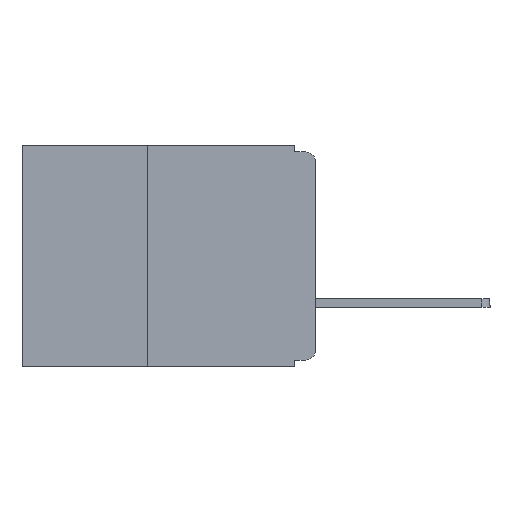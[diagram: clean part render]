
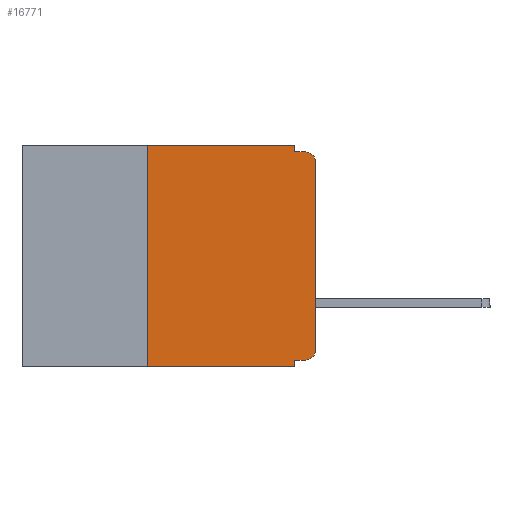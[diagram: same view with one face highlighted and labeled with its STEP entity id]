
A CAD part, left-side view. The second image highlights one B-rep face of the part: STEP entity #16771.
In plain terms, the highlighted planar face has unit normal (-1, 0, 0).
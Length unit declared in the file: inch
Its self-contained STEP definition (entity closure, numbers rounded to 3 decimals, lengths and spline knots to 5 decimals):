
#26 = PLANE ( 'NONE',  #10962 ) ;
#110 = CARTESIAN_POINT ( 'NONE',  ( 0., 0.437, 0. ) ) ;
#758 = ORIENTED_EDGE ( 'NONE', *, *, #4400, .T. ) ;
#957 = CARTESIAN_POINT ( 'NONE',  ( 0., 0., -0.305 ) ) ;
#1059 = CARTESIAN_POINT ( 'NONE',  ( 0., 0.031, 0. ) ) ;
#1191 = DIRECTION ( 'NONE',  ( 0., 0., -1. ) ) ;
#1295 = ORIENTED_EDGE ( 'NONE', *, *, #5879, .F. ) ;
#1357 = VERTEX_POINT ( 'NONE', #16873 ) ;
#1403 = VECTOR ( 'NONE', #18997, 39.37008 ) ;
#1561 = LINE ( 'NONE', #16957, #1403 ) ;
#1664 = VECTOR ( 'NONE', #6041, 39.37008 ) ;
#1813 = CARTESIAN_POINT ( 'NONE',  ( 0., 0.25, 0. ) ) ;
#1842 = LINE ( 'NONE', #18435, #1664 ) ;
#1916 = VERTEX_POINT ( 'NONE', #14373 ) ;
#2876 = VERTEX_POINT ( 'NONE', #17773 ) ;
#3123 = CARTESIAN_POINT ( 'NONE',  ( 0., 0.015, -0.32 ) ) ;
#3374 = DIRECTION ( 'NONE',  ( 0., 1., 0. ) ) ;
#3438 = CARTESIAN_POINT ( 'NONE',  ( 0., 0.25, -0.33 ) ) ;
#3558 = FACE_OUTER_BOUND ( 'NONE', #6465, .T. ) ;
#3839 = CARTESIAN_POINT ( 'NONE',  ( 0., 0., -0.32 ) ) ;
#3941 = CIRCLE ( 'NONE', #15819, 0.015 ) ;
#4025 = VECTOR ( 'NONE', #5223, 39.37008 ) ;
#4045 = LINE ( 'NONE', #4946, #4025 ) ;
#4400 = EDGE_CURVE ( 'NONE', #10610, #18652, #4756, .T. ) ;
#4712 = VECTOR ( 'NONE', #15009, 39.37008 ) ;
#4756 = LINE ( 'NONE', #14314, #4712 ) ;
#4854 = VECTOR ( 'NONE', #18071, 39.37008 ) ;
#4946 = CARTESIAN_POINT ( 'NONE',  ( 0., 0., -0.01 ) ) ;
#4978 = ORIENTED_EDGE ( 'NONE', *, *, #18513, .T. ) ;
#5032 = LINE ( 'NONE', #17976, #4854 ) ;
#5223 = DIRECTION ( 'NONE',  ( 0., -1., 0. ) ) ;
#5879 = EDGE_CURVE ( 'NONE', #12485, #2876, #12464, .T. ) ;
#6041 = DIRECTION ( 'NONE',  ( 0., -1., 0. ) ) ;
#6465 = EDGE_LOOP ( 'NONE', ( #758, #8889, #9563, #11610, #12666, #15090, #16672, #1295, #12717, #4978 ) ) ;
#7396 = VECTOR ( 'NONE', #3374, 39.37008 ) ;
#7537 = LINE ( 'NONE', #3839, #7396 ) ;
#7982 = CIRCLE ( 'NONE', #18578, 0.015 ) ;
#8578 = VECTOR ( 'NONE', #16058, 39.37008 ) ;
#8889 = ORIENTED_EDGE ( 'NONE', *, *, #14869, .T. ) ;
#9548 = DIRECTION ( 'NONE',  ( 0., 0., -1. ) ) ;
#9563 = ORIENTED_EDGE ( 'NONE', *, *, #11146, .F. ) ;
#9613 = DIRECTION ( 'NONE',  ( -1., 0., 0. ) ) ;
#9686 = CARTESIAN_POINT ( 'NONE',  ( 0., 0.015, -0.025 ) ) ;
#9831 = VERTEX_POINT ( 'NONE', #14413 ) ;
#10332 = EDGE_CURVE ( 'NONE', #17789, #2876, #1842, .T. ) ;
#10610 = VERTEX_POINT ( 'NONE', #957 ) ;
#10962 = AXIS2_PLACEMENT_3D ( 'NONE', #110, #19120, #19111 ) ;
#11146 = EDGE_CURVE ( 'NONE', #1357, #9831, #4045, .T. ) ;
#11537 = VERTEX_POINT ( 'NONE', #1813 ) ;
#11610 = ORIENTED_EDGE ( 'NONE', *, *, #17842, .F. ) ;
#11834 = CARTESIAN_POINT ( 'NONE',  ( 0., 0.031, -0.32 ) ) ;
#12326 = VECTOR ( 'NONE', #1191, 39.37008 ) ;
#12401 = LINE ( 'NONE', #1059, #12326 ) ;
#12464 = LINE ( 'NONE', #16303, #8578 ) ;
#12485 = VERTEX_POINT ( 'NONE', #11834 ) ;
#12666 = ORIENTED_EDGE ( 'NONE', *, *, #19063, .F. ) ;
#12717 = ORIENTED_EDGE ( 'NONE', *, *, #18622, .F. ) ;
#14314 = CARTESIAN_POINT ( 'NONE',  ( 0., 0., 0. ) ) ;
#14373 = CARTESIAN_POINT ( 'NONE',  ( 0., 0.031, 0. ) ) ;
#14413 = CARTESIAN_POINT ( 'NONE',  ( 0., 0.015, -0.01 ) ) ;
#14869 = EDGE_CURVE ( 'NONE', #18652, #9831, #3941, .T. ) ;
#15009 = DIRECTION ( 'NONE',  ( 0., 0., 1. ) ) ;
#15090 = ORIENTED_EDGE ( 'NONE', *, *, #17062, .F. ) ;
#15819 = AXIS2_PLACEMENT_3D ( 'NONE', #9686, #9613, #9548 ) ;
#15890 = DIRECTION ( 'NONE',  ( 0., 0., -1. ) ) ;
#16058 = DIRECTION ( 'NONE',  ( 0., 0., -1. ) ) ;
#16303 = CARTESIAN_POINT ( 'NONE',  ( 0., 0.031, -0.33 ) ) ;
#16672 = ORIENTED_EDGE ( 'NONE', *, *, #10332, .T. ) ;
#16714 = VERTEX_POINT ( 'NONE', #3123 ) ;
#16771 = ADVANCED_FACE ( 'NONE', ( #3558 ), #26, .F. ) ;
#16873 = CARTESIAN_POINT ( 'NONE',  ( 0., 0.031, -0.01 ) ) ;
#16939 = DIRECTION ( 'NONE',  ( -1., 0., 0. ) ) ;
#16957 = CARTESIAN_POINT ( 'NONE',  ( 0., 0.25, -0.33 ) ) ;
#16987 = CARTESIAN_POINT ( 'NONE',  ( 0., 0.015, -0.305 ) ) ;
#17062 = EDGE_CURVE ( 'NONE', #17789, #11537, #1561, .T. ) ;
#17773 = CARTESIAN_POINT ( 'NONE',  ( 0., 0.031, -0.33 ) ) ;
#17789 = VERTEX_POINT ( 'NONE', #3438 ) ;
#17842 = EDGE_CURVE ( 'NONE', #1916, #1357, #12401, .T. ) ;
#17976 = CARTESIAN_POINT ( 'NONE',  ( 0., 0.437, 0. ) ) ;
#18071 = DIRECTION ( 'NONE',  ( 0., -1., 0. ) ) ;
#18435 = CARTESIAN_POINT ( 'NONE',  ( 0., 0.437, -0.33 ) ) ;
#18513 = EDGE_CURVE ( 'NONE', #16714, #10610, #7982, .T. ) ;
#18578 = AXIS2_PLACEMENT_3D ( 'NONE', #16987, #16939, #15890 ) ;
#18622 = EDGE_CURVE ( 'NONE', #16714, #12485, #7537, .T. ) ;
#18652 = VERTEX_POINT ( 'NONE', #19157 ) ;
#18997 = DIRECTION ( 'NONE',  ( 0., 0., 1. ) ) ;
#19063 = EDGE_CURVE ( 'NONE', #11537, #1916, #5032, .T. ) ;
#19111 = DIRECTION ( 'NONE',  ( 0., 0., -1. ) ) ;
#19120 = DIRECTION ( 'NONE',  ( 1., 0., 0. ) ) ;
#19157 = CARTESIAN_POINT ( 'NONE',  ( 0., 0., -0.025 ) ) ;
